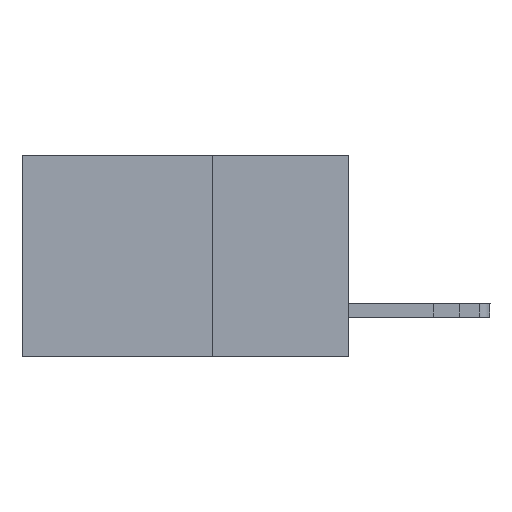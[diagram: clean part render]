
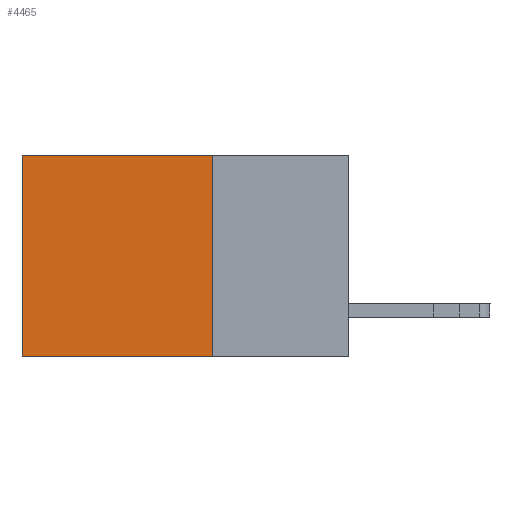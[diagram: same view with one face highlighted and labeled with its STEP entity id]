
A CAD part, left-side view. The second image highlights one B-rep face of the part: STEP entity #4465.
In plain terms, the highlighted planar face has unit normal (-1, 0, 0).
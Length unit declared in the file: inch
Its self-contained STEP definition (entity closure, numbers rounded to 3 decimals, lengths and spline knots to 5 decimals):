
#363 = DIRECTION ( 'NONE',  ( 0., 0., -1. ) ) ;
#1080 = VECTOR ( 'NONE', #1174, 39.37008 ) ;
#1112 = CARTESIAN_POINT ( 'NONE',  ( 0.2615, 0.25, 0. ) ) ;
#1174 = DIRECTION ( 'NONE',  ( 0., 1., 0. ) ) ;
#1850 = CARTESIAN_POINT ( 'NONE',  ( 0.2615, 0.25, -0.37 ) ) ;
#2705 = CARTESIAN_POINT ( 'NONE',  ( 0.2615, 0.25, 0. ) ) ;
#3564 = VERTEX_POINT ( 'NONE', #4044 ) ;
#4044 = CARTESIAN_POINT ( 'NONE',  ( 0.2615, 0.6, -0.37 ) ) ;
#4465 = ADVANCED_FACE ( 'NONE', ( #10051 ), #5744, .F. ) ;
#4544 = CARTESIAN_POINT ( 'NONE',  ( 0.2615, 0.6, 0. ) ) ;
#4868 = VECTOR ( 'NONE', #363, 39.37008 ) ;
#4965 = CARTESIAN_POINT ( 'NONE',  ( 0.2615, 0.25, -0.37 ) ) ;
#5494 = CARTESIAN_POINT ( 'NONE',  ( 0.2615, 0.25, -0.37 ) ) ;
#5744 = PLANE ( 'NONE',  #8966 ) ;
#5867 = DIRECTION ( 'NONE',  ( 0., 1., 0. ) ) ;
#6143 = EDGE_CURVE ( 'NONE', #9596, #7169, #9498, .T. ) ;
#6269 = VECTOR ( 'NONE', #5867, 39.37008 ) ;
#6382 = EDGE_CURVE ( 'NONE', #7169, #3564, #10775, .T. ) ;
#6633 = ORIENTED_EDGE ( 'NONE', *, *, #6143, .T. ) ;
#6760 = VECTOR ( 'NONE', #10887, 39.37008 ) ;
#6912 = LINE ( 'NONE', #1850, #6269 ) ;
#6932 = VERTEX_POINT ( 'NONE', #7800 ) ;
#6986 = ORIENTED_EDGE ( 'NONE', *, *, #10557, .F. ) ;
#7169 = VERTEX_POINT ( 'NONE', #4544 ) ;
#7514 = CARTESIAN_POINT ( 'NONE',  ( 0.2615, 0.6, -0.37 ) ) ;
#7800 = CARTESIAN_POINT ( 'NONE',  ( 0.2615, 0.25, -0.37 ) ) ;
#8189 = DIRECTION ( 'NONE',  ( 1., 0., 0. ) ) ;
#8509 = EDGE_LOOP ( 'NONE', ( #10271, #10116, #6986, #6633 ) ) ;
#8966 = AXIS2_PLACEMENT_3D ( 'NONE', #4965, #8189, #9214 ) ;
#9214 = DIRECTION ( 'NONE',  ( 0., 0., -1. ) ) ;
#9498 = LINE ( 'NONE', #1112, #1080 ) ;
#9596 = VERTEX_POINT ( 'NONE', #2705 ) ;
#10051 = FACE_OUTER_BOUND ( 'NONE', #8509, .T. ) ;
#10116 = ORIENTED_EDGE ( 'NONE', *, *, #10413, .F. ) ;
#10271 = ORIENTED_EDGE ( 'NONE', *, *, #6382, .T. ) ;
#10413 = EDGE_CURVE ( 'NONE', #6932, #3564, #6912, .T. ) ;
#10557 = EDGE_CURVE ( 'NONE', #9596, #6932, #10562, .T. ) ;
#10562 = LINE ( 'NONE', #5494, #4868 ) ;
#10775 = LINE ( 'NONE', #7514, #6760 ) ;
#10887 = DIRECTION ( 'NONE',  ( 0., 0., -1. ) ) ;
